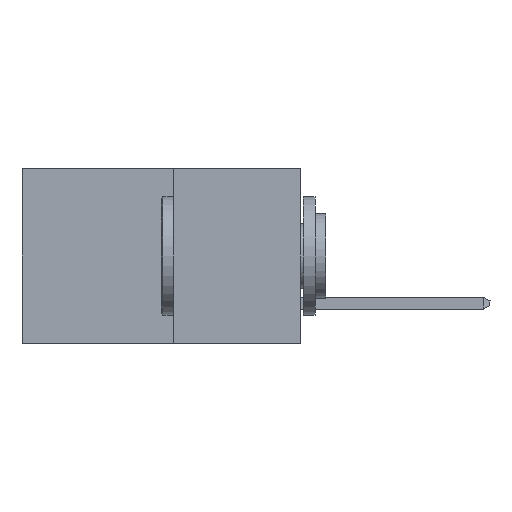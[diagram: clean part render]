
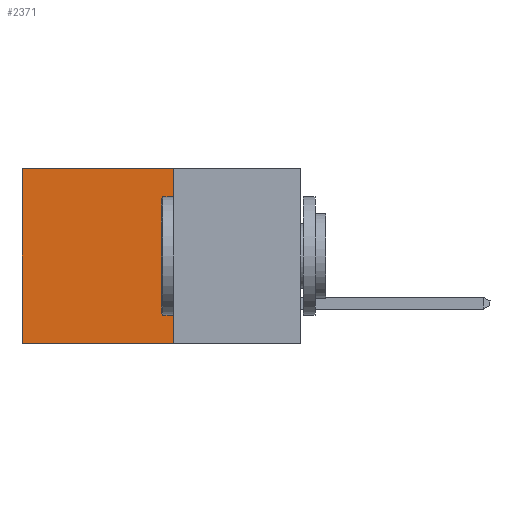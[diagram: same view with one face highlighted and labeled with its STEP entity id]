
A CAD part, left-side view. The second image highlights one B-rep face of the part: STEP entity #2371.
In plain terms, the highlighted planar face has unit normal (-1, 0, 0).
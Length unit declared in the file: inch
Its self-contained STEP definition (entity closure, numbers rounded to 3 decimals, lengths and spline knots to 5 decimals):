
#346 = VERTEX_POINT ( 'NONE', #6458 ) ;
#359 = EDGE_CURVE ( 'NONE', #346, #8574, #6347, .T. ) ;
#740 = EDGE_CURVE ( 'NONE', #8915, #3136, #4690, .T. ) ;
#1948 = CARTESIAN_POINT ( 'NONE',  ( 0.277, 0.59, -0.37 ) ) ;
#2300 = EDGE_CURVE ( 'NONE', #8574, #3136, #3668, .T. ) ;
#2371 = ADVANCED_FACE ( 'NONE', ( #6552 ), #3893, .F. ) ;
#2457 = DIRECTION ( 'NONE',  ( 1., 0., 0. ) ) ;
#2820 = CARTESIAN_POINT ( 'NONE',  ( 0.277, 0.27, -0.37 ) ) ;
#2873 = VECTOR ( 'NONE', #6405, 39.37008 ) ;
#3136 = VERTEX_POINT ( 'NONE', #1948 ) ;
#3668 = LINE ( 'NONE', #6498, #7453 ) ;
#3802 = DIRECTION ( 'NONE',  ( 0., 0., -1. ) ) ;
#3893 = PLANE ( 'NONE',  #4119 ) ;
#4119 = AXIS2_PLACEMENT_3D ( 'NONE', #4381, #2457, #3802 ) ;
#4381 = CARTESIAN_POINT ( 'NONE',  ( 0.277, 0.27, -0.37 ) ) ;
#4690 = LINE ( 'NONE', #8628, #8572 ) ;
#4722 = CARTESIAN_POINT ( 'NONE',  ( 0.277, 0.27, -0.37 ) ) ;
#4898 = CARTESIAN_POINT ( 'NONE',  ( 0.277, 0.27, 0. ) ) ;
#5731 = ORIENTED_EDGE ( 'NONE', *, *, #7743, .T. ) ;
#5921 = DIRECTION ( 'NONE',  ( 0., 0., -1. ) ) ;
#6297 = ORIENTED_EDGE ( 'NONE', *, *, #359, .F. ) ;
#6347 = LINE ( 'NONE', #2820, #7817 ) ;
#6405 = DIRECTION ( 'NONE',  ( 0., 1., 0. ) ) ;
#6458 = CARTESIAN_POINT ( 'NONE',  ( 0.277, 0.27, 0. ) ) ;
#6498 = CARTESIAN_POINT ( 'NONE',  ( 0.277, 0.27, -0.37 ) ) ;
#6552 = FACE_OUTER_BOUND ( 'NONE', #9319, .T. ) ;
#6933 = LINE ( 'NONE', #4898, #2873 ) ;
#7333 = ORIENTED_EDGE ( 'NONE', *, *, #2300, .F. ) ;
#7453 = VECTOR ( 'NONE', #8385, 39.37008 ) ;
#7465 = ORIENTED_EDGE ( 'NONE', *, *, #740, .T. ) ;
#7743 = EDGE_CURVE ( 'NONE', #346, #8915, #6933, .T. ) ;
#7817 = VECTOR ( 'NONE', #5921, 39.37008 ) ;
#8385 = DIRECTION ( 'NONE',  ( 0., 1., 0. ) ) ;
#8572 = VECTOR ( 'NONE', #8630, 39.37008 ) ;
#8574 = VERTEX_POINT ( 'NONE', #4722 ) ;
#8628 = CARTESIAN_POINT ( 'NONE',  ( 0.277, 0.59, -0.37 ) ) ;
#8630 = DIRECTION ( 'NONE',  ( 0., 0., -1. ) ) ;
#8915 = VERTEX_POINT ( 'NONE', #9260 ) ;
#9260 = CARTESIAN_POINT ( 'NONE',  ( 0.277, 0.59, 0. ) ) ;
#9319 = EDGE_LOOP ( 'NONE', ( #7465, #7333, #6297, #5731 ) ) ;
